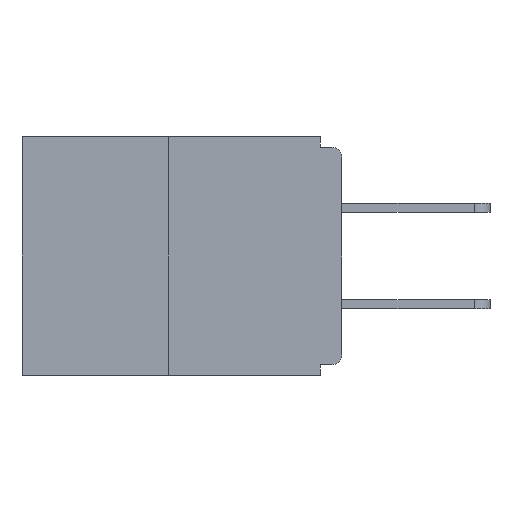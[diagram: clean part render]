
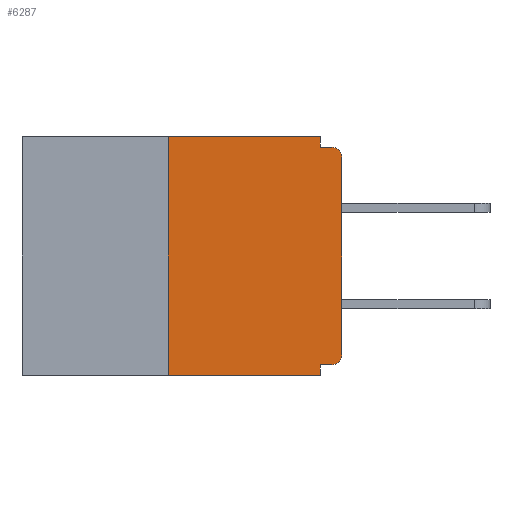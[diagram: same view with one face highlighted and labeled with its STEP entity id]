
A CAD part, left-side view. The second image highlights one B-rep face of the part: STEP entity #6287.
In plain terms, the highlighted planar face has unit normal (-1, 0, 0).
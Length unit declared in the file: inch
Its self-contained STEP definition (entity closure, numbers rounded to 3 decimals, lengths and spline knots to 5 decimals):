
#261 = EDGE_CURVE ( 'NONE', #8246, #10441, #1546, .T. ) ;
#282 = CARTESIAN_POINT ( 'NONE',  ( 0., 0.031, 0. ) ) ;
#289 = DIRECTION ( 'NONE',  ( 0., 0., -1. ) ) ;
#372 = DIRECTION ( 'NONE',  ( 0., -1., 0. ) ) ;
#1335 = CARTESIAN_POINT ( 'NONE',  ( 0., 0.031, 0. ) ) ;
#1476 = EDGE_LOOP ( 'NONE', ( #3893, #8977, #4250, #5421, #3892, #4918, #2686, #3215, #7030, #3086 ) ) ;
#1546 = CIRCLE ( 'NONE', #8698, 0.015 ) ;
#1732 = VERTEX_POINT ( 'NONE', #4232 ) ;
#1765 = CARTESIAN_POINT ( 'NONE',  ( 0., 0.031, -0.328 ) ) ;
#1856 = LINE ( 'NONE', #9080, #5677 ) ;
#1924 = LINE ( 'NONE', #282, #9959 ) ;
#1976 = PLANE ( 'NONE',  #9478 ) ;
#2025 = LINE ( 'NONE', #3628, #9387 ) ;
#2105 = CARTESIAN_POINT ( 'NONE',  ( 0., 0.46, 0. ) ) ;
#2282 = VERTEX_POINT ( 'NONE', #4348 ) ;
#2321 = VECTOR ( 'NONE', #372, 39.37008 ) ;
#2354 = EDGE_CURVE ( 'NONE', #5960, #10441, #9429, .T. ) ;
#2423 = EDGE_CURVE ( 'NONE', #6341, #5960, #1924, .T. ) ;
#2613 = DIRECTION ( 'NONE',  ( -1., 0., 0. ) ) ;
#2686 = ORIENTED_EDGE ( 'NONE', *, *, #6833, .T. ) ;
#2730 = EDGE_CURVE ( 'NONE', #4409, #4050, #9550, .T. ) ;
#2747 = DIRECTION ( 'NONE',  ( 1., 0., 0. ) ) ;
#2777 = DIRECTION ( 'NONE',  ( 0., -1., 0. ) ) ;
#2872 = CARTESIAN_POINT ( 'NONE',  ( 0., 0.46, 0. ) ) ;
#3086 = ORIENTED_EDGE ( 'NONE', *, *, #2423, .F. ) ;
#3215 = ORIENTED_EDGE ( 'NONE', *, *, #261, .T. ) ;
#3269 = EDGE_CURVE ( 'NONE', #2282, #4050, #7823, .T. ) ;
#3578 = CARTESIAN_POINT ( 'NONE',  ( 0., 0., -0.015 ) ) ;
#3628 = CARTESIAN_POINT ( 'NONE',  ( 0., 0., -0.328 ) ) ;
#3632 = EDGE_CURVE ( 'NONE', #2282, #10156, #1856, .T. ) ;
#3855 = CARTESIAN_POINT ( 'NONE',  ( 0., 0.031, -0.015 ) ) ;
#3861 = DIRECTION ( 'NONE',  ( 0., 0., 1. ) ) ;
#3892 = ORIENTED_EDGE ( 'NONE', *, *, #8566, .F. ) ;
#3893 = ORIENTED_EDGE ( 'NONE', *, *, #10330, .F. ) ;
#4050 = VERTEX_POINT ( 'NONE', #4507 ) ;
#4089 = DIRECTION ( 'NONE',  ( -1., 0., 0. ) ) ;
#4232 = CARTESIAN_POINT ( 'NONE',  ( 0., 0.015, -0.328 ) ) ;
#4250 = ORIENTED_EDGE ( 'NONE', *, *, #3269, .T. ) ;
#4348 = CARTESIAN_POINT ( 'NONE',  ( 0., 0.25, -0.343 ) ) ;
#4409 = VERTEX_POINT ( 'NONE', #1765 ) ;
#4411 = CARTESIAN_POINT ( 'NONE',  ( 0., 0.25, 0. ) ) ;
#4507 = CARTESIAN_POINT ( 'NONE',  ( 0., 0.031, -0.343 ) ) ;
#4625 = LINE ( 'NONE', #2105, #2321 ) ;
#4703 = VERTEX_POINT ( 'NONE', #9938 ) ;
#4874 = CARTESIAN_POINT ( 'NONE',  ( 0., 0.46, -0.343 ) ) ;
#4913 = CARTESIAN_POINT ( 'NONE',  ( 0., 0.031, -0.343 ) ) ;
#4918 = ORIENTED_EDGE ( 'NONE', *, *, #10517, .T. ) ;
#4958 = CARTESIAN_POINT ( 'NONE',  ( 0., 0.015, -0.03 ) ) ;
#5228 = DIRECTION ( 'NONE',  ( 0., 1., 0. ) ) ;
#5348 = VECTOR ( 'NONE', #2777, 39.37008 ) ;
#5421 = ORIENTED_EDGE ( 'NONE', *, *, #2730, .F. ) ;
#5677 = VECTOR ( 'NONE', #3861, 39.37008 ) ;
#5729 = AXIS2_PLACEMENT_3D ( 'NONE', #10492, #2613, #7877 ) ;
#5879 = FACE_OUTER_BOUND ( 'NONE', #1476, .T. ) ;
#5960 = VERTEX_POINT ( 'NONE', #3855 ) ;
#6287 = ADVANCED_FACE ( 'NONE', ( #5879 ), #1976, .F. ) ;
#6291 = VECTOR ( 'NONE', #8338, 39.37008 ) ;
#6341 = VERTEX_POINT ( 'NONE', #1335 ) ;
#6464 = CARTESIAN_POINT ( 'NONE',  ( 0., 0., 0. ) ) ;
#6709 = VECTOR ( 'NONE', #10855, 39.37008 ) ;
#6833 = EDGE_CURVE ( 'NONE', #4703, #8246, #6956, .T. ) ;
#6956 = LINE ( 'NONE', #6464, #6291 ) ;
#7030 = ORIENTED_EDGE ( 'NONE', *, *, #2354, .F. ) ;
#7823 = LINE ( 'NONE', #4874, #7969 ) ;
#7877 = DIRECTION ( 'NONE',  ( 0., 0., -1. ) ) ;
#7969 = VECTOR ( 'NONE', #9206, 39.37008 ) ;
#8246 = VERTEX_POINT ( 'NONE', #10043 ) ;
#8338 = DIRECTION ( 'NONE',  ( 0., 0., 1. ) ) ;
#8566 = EDGE_CURVE ( 'NONE', #1732, #4409, #2025, .T. ) ;
#8698 = AXIS2_PLACEMENT_3D ( 'NONE', #4958, #4089, #10147 ) ;
#8977 = ORIENTED_EDGE ( 'NONE', *, *, #3632, .F. ) ;
#9080 = CARTESIAN_POINT ( 'NONE',  ( 0., 0.25, 0. ) ) ;
#9206 = DIRECTION ( 'NONE',  ( 0., -1., 0. ) ) ;
#9226 = CARTESIAN_POINT ( 'NONE',  ( 0., 0.015, -0.015 ) ) ;
#9251 = CIRCLE ( 'NONE', #5729, 0.015 ) ;
#9387 = VECTOR ( 'NONE', #5228, 39.37008 ) ;
#9429 = LINE ( 'NONE', #3578, #5348 ) ;
#9478 = AXIS2_PLACEMENT_3D ( 'NONE', #2872, #2747, #289 ) ;
#9550 = LINE ( 'NONE', #4913, #6709 ) ;
#9623 = DIRECTION ( 'NONE',  ( 0., 0., -1. ) ) ;
#9938 = CARTESIAN_POINT ( 'NONE',  ( 0., 0., -0.313 ) ) ;
#9959 = VECTOR ( 'NONE', #9623, 39.37008 ) ;
#10043 = CARTESIAN_POINT ( 'NONE',  ( 0., 0., -0.03 ) ) ;
#10147 = DIRECTION ( 'NONE',  ( 0., 0., -1. ) ) ;
#10156 = VERTEX_POINT ( 'NONE', #4411 ) ;
#10330 = EDGE_CURVE ( 'NONE', #10156, #6341, #4625, .T. ) ;
#10441 = VERTEX_POINT ( 'NONE', #9226 ) ;
#10492 = CARTESIAN_POINT ( 'NONE',  ( 0., 0.015, -0.313 ) ) ;
#10517 = EDGE_CURVE ( 'NONE', #1732, #4703, #9251, .T. ) ;
#10855 = DIRECTION ( 'NONE',  ( 0., 0., -1. ) ) ;
